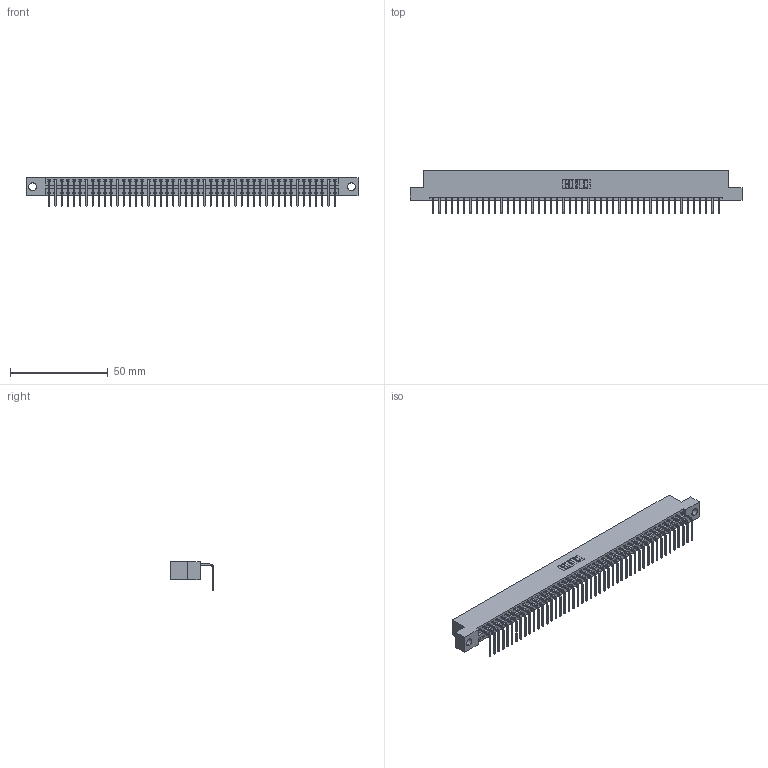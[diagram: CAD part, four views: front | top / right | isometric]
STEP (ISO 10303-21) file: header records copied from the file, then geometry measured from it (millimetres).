
FILE_DESCRIPTION (( 'STEP AP203' ), '1' );
FILE_NAME ('396-047-558-104.STEP', '2019-11-01T08:22:12', ( '' ), ( '' ), 'SwSTEP 2.0', 'SolidWorks 2016', '' );
FILE_SCHEMA (( 'CONFIG_CONTROL_DESIGN' ));
Length unit declared in the file: inch
Products named in the file (3): 346 Part_Flush Mounting Lugs - 0.156 Dia-TH; 345-292-001_558 Tail - 2; 396-047-558-104
Assembly tree (48 placements, depth 2):
  396-047-558-104
    346 Part_Flush Mounting Lugs - 0.156 Dia-TH
    345-292-001_558 Tail - 2  x47
Bounding box: 169.8 x 22.16 x 14.73 mm (x, y, z)
Volume: 16356.7 mm3; surface area: 21236.9 mm2
Topology: 48 solids, 48 shells, 2942 faces, 8883 edges, 5858 vertices
Faces by surface type: plane 2050, cylinder 892
Entity records: 28583 total; most frequent: CARTESIAN_POINT 4905, ORIENTED_EDGE 4886, DIRECTION 4321, EDGE_CURVE 2443, LINE 2123, VECTOR 2123, VERTEX_POINT 1626, AXIS2_PLACEMENT_3D 1099
